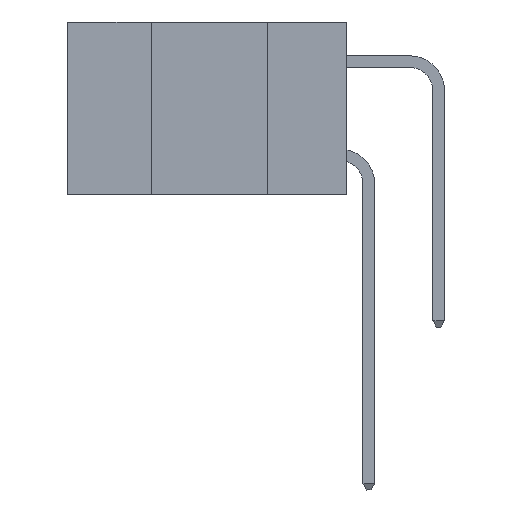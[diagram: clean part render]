
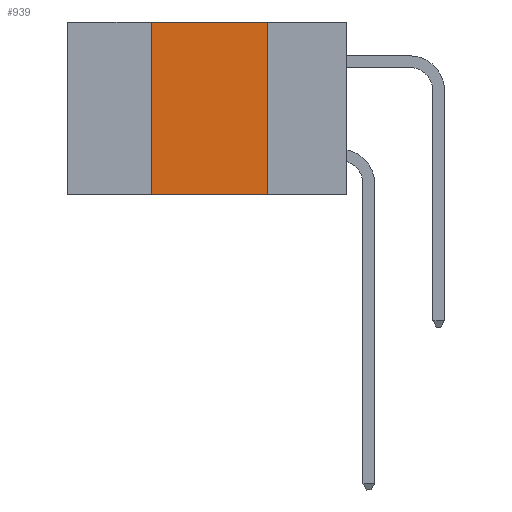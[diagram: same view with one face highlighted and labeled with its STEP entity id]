
A CAD part, left-side view. The second image highlights one B-rep face of the part: STEP entity #939.
In plain terms, the highlighted planar face has unit normal (-1, 0, 0).
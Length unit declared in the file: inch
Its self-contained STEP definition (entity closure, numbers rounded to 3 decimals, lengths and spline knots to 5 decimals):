
#473 = CARTESIAN_POINT ( 'NONE',  ( 0., 0.17, 0. ) ) ;
#939 = ADVANCED_FACE ( 'NONE', ( #17184 ), #17654, .F. ) ;
#3470 = VERTEX_POINT ( 'NONE', #22400 ) ;
#3999 = LINE ( 'NONE', #22868, #22788 ) ;
#5325 = LINE ( 'NONE', #9927, #19757 ) ;
#5750 = CARTESIAN_POINT ( 'NONE',  ( 0., 0.42, 0. ) ) ;
#5945 = DIRECTION ( 'NONE',  ( 1., 0., 0. ) ) ;
#9927 = CARTESIAN_POINT ( 'NONE',  ( 0., 0.6, 0. ) ) ;
#10194 = VECTOR ( 'NONE', #19072, 39.37008 ) ;
#10409 = CARTESIAN_POINT ( 'NONE',  ( 0., 0.17, 0. ) ) ;
#11587 = ORIENTED_EDGE ( 'NONE', *, *, #13746, .T. ) ;
#11664 = CARTESIAN_POINT ( 'NONE',  ( 0., 0.6, -0.37 ) ) ;
#11885 = DIRECTION ( 'NONE',  ( 0., -1., 0. ) ) ;
#12065 = DIRECTION ( 'NONE',  ( 0., 0., -1. ) ) ;
#13672 = DIRECTION ( 'NONE',  ( 0., 0., 1. ) ) ;
#13746 = EDGE_CURVE ( 'NONE', #3470, #21246, #14657, .T. ) ;
#13844 = EDGE_LOOP ( 'NONE', ( #19918, #19703, #20007, #11587 ) ) ;
#13942 = AXIS2_PLACEMENT_3D ( 'NONE', #16381, #5945, #12065 ) ;
#14657 = LINE ( 'NONE', #11664, #10194 ) ;
#14709 = LINE ( 'NONE', #473, #19049 ) ;
#15897 = VERTEX_POINT ( 'NONE', #5750 ) ;
#16381 = CARTESIAN_POINT ( 'NONE',  ( 0., 0.6, 0. ) ) ;
#17184 = FACE_OUTER_BOUND ( 'NONE', #13844, .T. ) ;
#17654 = PLANE ( 'NONE',  #13942 ) ;
#17836 = EDGE_CURVE ( 'NONE', #3470, #15897, #3999, .T. ) ;
#19049 = VECTOR ( 'NONE', #21151, 39.37008 ) ;
#19072 = DIRECTION ( 'NONE',  ( 0., -1., 0. ) ) ;
#19703 = ORIENTED_EDGE ( 'NONE', *, *, #22999, .F. ) ;
#19757 = VECTOR ( 'NONE', #11885, 39.37008 ) ;
#19918 = ORIENTED_EDGE ( 'NONE', *, *, #20311, .F. ) ;
#20007 = ORIENTED_EDGE ( 'NONE', *, *, #17836, .F. ) ;
#20311 = EDGE_CURVE ( 'NONE', #23859, #21246, #14709, .T. ) ;
#20972 = CARTESIAN_POINT ( 'NONE',  ( 0., 0.17, -0.37 ) ) ;
#21151 = DIRECTION ( 'NONE',  ( 0., 0., -1. ) ) ;
#21246 = VERTEX_POINT ( 'NONE', #20972 ) ;
#22400 = CARTESIAN_POINT ( 'NONE',  ( 0., 0.42, -0.37 ) ) ;
#22788 = VECTOR ( 'NONE', #13672, 39.37008 ) ;
#22868 = CARTESIAN_POINT ( 'NONE',  ( 0., 0.42, 0. ) ) ;
#22999 = EDGE_CURVE ( 'NONE', #15897, #23859, #5325, .T. ) ;
#23859 = VERTEX_POINT ( 'NONE', #10409 ) ;
